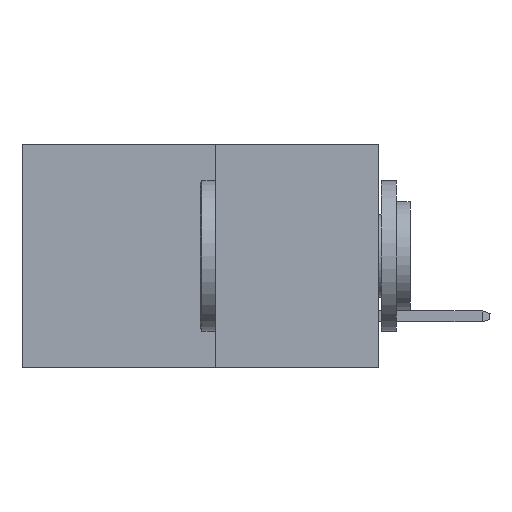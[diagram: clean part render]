
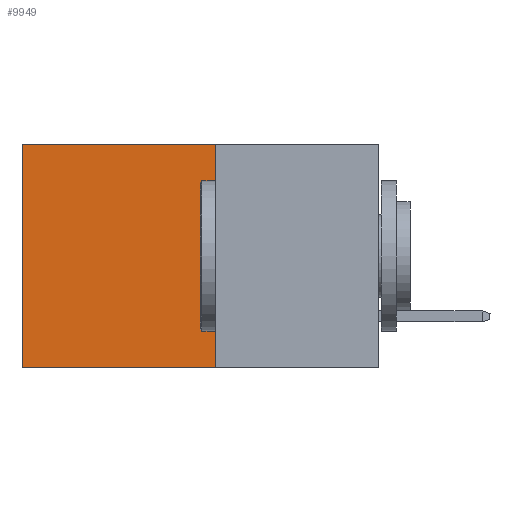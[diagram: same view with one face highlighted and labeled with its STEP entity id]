
A CAD part, left-side view. The second image highlights one B-rep face of the part: STEP entity #9949.
In plain terms, the highlighted planar face has unit normal (-1, 0, 0).
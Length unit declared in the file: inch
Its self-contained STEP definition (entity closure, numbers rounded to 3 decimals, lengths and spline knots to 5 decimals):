
#26 = EDGE_CURVE ( 'NONE', #3344, #8933, #1724, .T. ) ;
#175 = CARTESIAN_POINT ( 'NONE',  ( 0.277, 0.27, -0.37 ) ) ;
#346 = CARTESIAN_POINT ( 'NONE',  ( 0.277, 0.59, -0.37 ) ) ;
#1070 = DIRECTION ( 'NONE',  ( 0., 0., -1. ) ) ;
#1724 = LINE ( 'NONE', #175, #3755 ) ;
#1972 = EDGE_CURVE ( 'NONE', #3344, #3462, #7883, .T. ) ;
#2047 = AXIS2_PLACEMENT_3D ( 'NONE', #6282, #6315, #1070 ) ;
#2162 = ORIENTED_EDGE ( 'NONE', *, *, #4473, .F. ) ;
#2374 = ORIENTED_EDGE ( 'NONE', *, *, #1972, .T. ) ;
#2535 = ORIENTED_EDGE ( 'NONE', *, *, #26, .F. ) ;
#2821 = ORIENTED_EDGE ( 'NONE', *, *, #2977, .T. ) ;
#2845 = LINE ( 'NONE', #6040, #3116 ) ;
#2929 = PLANE ( 'NONE',  #2047 ) ;
#2977 = EDGE_CURVE ( 'NONE', #3462, #5814, #9210, .T. ) ;
#3116 = VECTOR ( 'NONE', #5931, 39.37008 ) ;
#3344 = VERTEX_POINT ( 'NONE', #10232 ) ;
#3462 = VERTEX_POINT ( 'NONE', #7204 ) ;
#3552 = VECTOR ( 'NONE', #8093, 39.37008 ) ;
#3755 = VECTOR ( 'NONE', #7482, 39.37008 ) ;
#4473 = EDGE_CURVE ( 'NONE', #8933, #5814, #2845, .T. ) ;
#4996 = VECTOR ( 'NONE', #9060, 39.37008 ) ;
#5814 = VERTEX_POINT ( 'NONE', #346 ) ;
#5931 = DIRECTION ( 'NONE',  ( 0., 1., 0. ) ) ;
#6002 = CARTESIAN_POINT ( 'NONE',  ( 0.277, 0.27, -0.37 ) ) ;
#6040 = CARTESIAN_POINT ( 'NONE',  ( 0.277, 0.27, -0.37 ) ) ;
#6282 = CARTESIAN_POINT ( 'NONE',  ( 0.277, 0.27, -0.37 ) ) ;
#6315 = DIRECTION ( 'NONE',  ( 1., 0., 0. ) ) ;
#6671 = FACE_OUTER_BOUND ( 'NONE', #6930, .T. ) ;
#6930 = EDGE_LOOP ( 'NONE', ( #2821, #2162, #2535, #2374 ) ) ;
#7204 = CARTESIAN_POINT ( 'NONE',  ( 0.277, 0.59, 0. ) ) ;
#7482 = DIRECTION ( 'NONE',  ( 0., 0., -1. ) ) ;
#7883 = LINE ( 'NONE', #8069, #3552 ) ;
#8069 = CARTESIAN_POINT ( 'NONE',  ( 0.277, 0.27, 0. ) ) ;
#8093 = DIRECTION ( 'NONE',  ( 0., 1., 0. ) ) ;
#8108 = CARTESIAN_POINT ( 'NONE',  ( 0.277, 0.59, -0.37 ) ) ;
#8933 = VERTEX_POINT ( 'NONE', #6002 ) ;
#9060 = DIRECTION ( 'NONE',  ( 0., 0., -1. ) ) ;
#9210 = LINE ( 'NONE', #8108, #4996 ) ;
#9949 = ADVANCED_FACE ( 'NONE', ( #6671 ), #2929, .F. ) ;
#10232 = CARTESIAN_POINT ( 'NONE',  ( 0.277, 0.27, 0. ) ) ;
